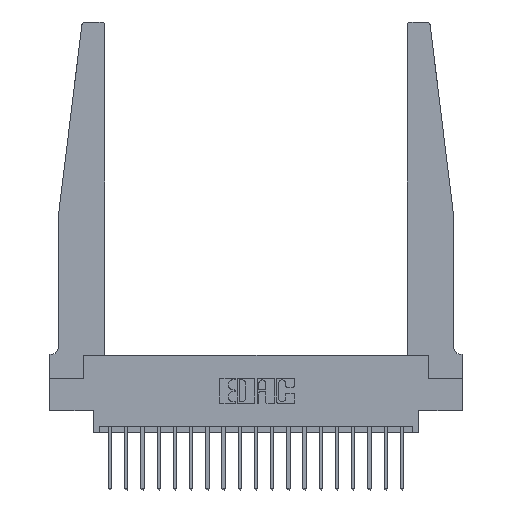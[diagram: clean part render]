
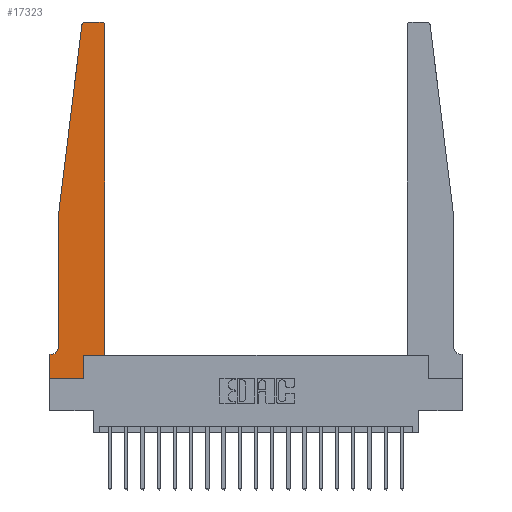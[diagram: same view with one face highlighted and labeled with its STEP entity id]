
A CAD part, top view. The second image highlights one B-rep face of the part: STEP entity #17323.
In plain terms, the highlighted planar face has unit normal (0, 0, 1).
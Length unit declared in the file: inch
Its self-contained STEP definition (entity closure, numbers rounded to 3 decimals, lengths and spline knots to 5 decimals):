
#47 = CARTESIAN_POINT ( 'NONE',  ( 0.2605, 0.18, 0.37 ) ) ;
#132 = VECTOR ( 'NONE', #20609, 39.37008 ) ;
#240 = LINE ( 'NONE', #17672, #7731 ) ;
#1497 = ORIENTED_EDGE ( 'NONE', *, *, #16786, .T. ) ;
#1586 = EDGE_CURVE ( 'NONE', #15586, #9109, #5750, .T. ) ;
#1587 = CARTESIAN_POINT ( 'NONE',  ( 0.27653, 2.72, 0.37 ) ) ;
#2582 = CARTESIAN_POINT ( 'NONE',  ( 0.065, 1.25, 0.37 ) ) ;
#2878 = VERTEX_POINT ( 'NONE', #9176 ) ;
#3000 = VERTEX_POINT ( 'NONE', #47 ) ;
#3519 = VECTOR ( 'NONE', #15939, 39.37008 ) ;
#3667 = CARTESIAN_POINT ( 'NONE',  ( 0.425, 2.72, 0.37 ) ) ;
#3804 = EDGE_CURVE ( 'NONE', #12323, #13643, #16821, .T. ) ;
#4185 = DIRECTION ( 'NONE',  ( 0., -1., 0. ) ) ;
#4323 = AXIS2_PLACEMENT_3D ( 'NONE', #16338, #6846, #18126 ) ;
#4395 = LINE ( 'NONE', #7848, #6207 ) ;
#4576 = VECTOR ( 'NONE', #19691, 39.37008 ) ;
#5034 = VECTOR ( 'NONE', #5542, 39.37008 ) ;
#5292 = ORIENTED_EDGE ( 'NONE', *, *, #1586, .T. ) ;
#5542 = DIRECTION ( 'NONE',  ( -0.122, -0.992, 0. ) ) ;
#5750 = CIRCLE ( 'NONE', #15189, 0.03 ) ;
#6018 = FACE_OUTER_BOUND ( 'NONE', #18411, .T. ) ;
#6207 = VECTOR ( 'NONE', #20681, 39.37008 ) ;
#6268 = ORIENTED_EDGE ( 'NONE', *, *, #15083, .T. ) ;
#6432 = EDGE_CURVE ( 'NONE', #2878, #19198, #14744, .T. ) ;
#6476 = CIRCLE ( 'NONE', #10875, 0.03 ) ;
#6534 = CARTESIAN_POINT ( 'NONE',  ( 0.425, 0.18, 0.37 ) ) ;
#6609 = DIRECTION ( 'NONE',  ( -1., 0., 0. ) ) ;
#6846 = DIRECTION ( 'NONE',  ( 0., 0., -1. ) ) ;
#6865 = LINE ( 'NONE', #19290, #10274 ) ;
#6880 = EDGE_CURVE ( 'NONE', #9109, #13700, #240, .T. ) ;
#6904 = EDGE_CURVE ( 'NONE', #13643, #2878, #16839, .T. ) ;
#6980 = CARTESIAN_POINT ( 'NONE',  ( 0., 0., 0.37 ) ) ;
#7018 = ORIENTED_EDGE ( 'NONE', *, *, #18342, .T. ) ;
#7120 = CARTESIAN_POINT ( 'NONE',  ( 0.065, 1.25, 0.37 ) ) ;
#7731 = VECTOR ( 'NONE', #6609, 39.37008 ) ;
#7848 = CARTESIAN_POINT ( 'NONE',  ( 0.2605, 0.18, 0.37 ) ) ;
#8049 = DIRECTION ( 'NONE',  ( 0., 0., 1. ) ) ;
#8143 = LINE ( 'NONE', #13001, #132 ) ;
#8332 = CARTESIAN_POINT ( 'NONE',  ( 0.395, 2.72, 0.37 ) ) ;
#8699 = ORIENTED_EDGE ( 'NONE', *, *, #3804, .T. ) ;
#8808 = EDGE_CURVE ( 'NONE', #13700, #12323, #6476, .T. ) ;
#8910 = CARTESIAN_POINT ( 'NONE',  ( 0.065, 1.25, 0.37 ) ) ;
#9109 = VERTEX_POINT ( 'NONE', #15541 ) ;
#9176 = CARTESIAN_POINT ( 'NONE',  ( 0.065, 0.2375, 0.37 ) ) ;
#9269 = CARTESIAN_POINT ( 'NONE',  ( 0., 0.1875, 0.37 ) ) ;
#9501 = CARTESIAN_POINT ( 'NONE',  ( 0.425, 0.18, 0.37 ) ) ;
#9592 = LINE ( 'NONE', #9501, #3519 ) ;
#10148 = DIRECTION ( 'NONE',  ( 0., -1., 0. ) ) ;
#10180 = ORIENTED_EDGE ( 'NONE', *, *, #8808, .T. ) ;
#10274 = VECTOR ( 'NONE', #14686, 39.37008 ) ;
#10875 = AXIS2_PLACEMENT_3D ( 'NONE', #1587, #8049, #11531 ) ;
#10895 = CARTESIAN_POINT ( 'NONE',  ( 0., 0., 0.37 ) ) ;
#11385 = EDGE_CURVE ( 'NONE', #3000, #20236, #19581, .T. ) ;
#11531 = DIRECTION ( 'NONE',  ( 1., 0., 0. ) ) ;
#11639 = VERTEX_POINT ( 'NONE', #12572 ) ;
#11799 = VECTOR ( 'NONE', #4185, 39.37008 ) ;
#11976 = ORIENTED_EDGE ( 'NONE', *, *, #16377, .T. ) ;
#12323 = VERTEX_POINT ( 'NONE', #19642 ) ;
#12463 = PLANE ( 'NONE',  #17398 ) ;
#12572 = CARTESIAN_POINT ( 'NONE',  ( 0., 0.1875, 0.37 ) ) ;
#12592 = ORIENTED_EDGE ( 'NONE', *, *, #11385, .T. ) ;
#13001 = CARTESIAN_POINT ( 'NONE',  ( 0., 0., 0.37 ) ) ;
#13522 = DIRECTION ( 'NONE',  ( 0., 0., 1. ) ) ;
#13526 = CARTESIAN_POINT ( 'NONE',  ( 0.2605, 0., 0.37 ) ) ;
#13643 = VERTEX_POINT ( 'NONE', #7120 ) ;
#13700 = VERTEX_POINT ( 'NONE', #15567 ) ;
#14534 = ORIENTED_EDGE ( 'NONE', *, *, #6432, .T. ) ;
#14686 = DIRECTION ( 'NONE',  ( -1., 0., 0. ) ) ;
#14744 = CIRCLE ( 'NONE', #4323, 0.05 ) ;
#14754 = CARTESIAN_POINT ( 'NONE',  ( 0.425, 0.18, 0.37 ) ) ;
#15083 = EDGE_CURVE ( 'NONE', #18611, #3000, #4395, .T. ) ;
#15189 = AXIS2_PLACEMENT_3D ( 'NONE', #8332, #13522, #18242 ) ;
#15541 = CARTESIAN_POINT ( 'NONE',  ( 0.395, 2.75, 0.37 ) ) ;
#15567 = CARTESIAN_POINT ( 'NONE',  ( 0.27653, 2.75, 0.37 ) ) ;
#15586 = VERTEX_POINT ( 'NONE', #3667 ) ;
#15939 = DIRECTION ( 'NONE',  ( 0., 1., 0. ) ) ;
#16329 = VECTOR ( 'NONE', #10148, 39.37008 ) ;
#16338 = CARTESIAN_POINT ( 'NONE',  ( 0.015, 0.2375, 0.37 ) ) ;
#16377 = EDGE_CURVE ( 'NONE', #18731, #18611, #8143, .T. ) ;
#16467 = EDGE_CURVE ( 'NONE', #11639, #18731, #18253, .T. ) ;
#16481 = ORIENTED_EDGE ( 'NONE', *, *, #16467, .T. ) ;
#16484 = ORIENTED_EDGE ( 'NONE', *, *, #6904, .T. ) ;
#16786 = EDGE_CURVE ( 'NONE', #20236, #15586, #9592, .T. ) ;
#16821 = LINE ( 'NONE', #8910, #5034 ) ;
#16839 = LINE ( 'NONE', #2582, #11799 ) ;
#17286 = CARTESIAN_POINT ( 'NONE',  ( 0.015, 0.1875, 0.37 ) ) ;
#17323 = ADVANCED_FACE ( 'NONE', ( #6018 ), #12463, .T. ) ;
#17391 = DIRECTION ( 'NONE',  ( 0., 0., 1. ) ) ;
#17398 = AXIS2_PLACEMENT_3D ( 'NONE', #9269, #17391, #20637 ) ;
#17672 = CARTESIAN_POINT ( 'NONE',  ( 0.25, 2.75, 0.37 ) ) ;
#18126 = DIRECTION ( 'NONE',  ( -1., 0., 0. ) ) ;
#18242 = DIRECTION ( 'NONE',  ( 1., 0., 0. ) ) ;
#18253 = LINE ( 'NONE', #6980, #16329 ) ;
#18342 = EDGE_CURVE ( 'NONE', #19198, #11639, #6865, .T. ) ;
#18411 = EDGE_LOOP ( 'NONE', ( #18706, #10180, #8699, #16484, #14534, #7018, #16481, #11976, #6268, #12592, #1497, #5292 ) ) ;
#18611 = VERTEX_POINT ( 'NONE', #13526 ) ;
#18706 = ORIENTED_EDGE ( 'NONE', *, *, #6880, .T. ) ;
#18731 = VERTEX_POINT ( 'NONE', #10895 ) ;
#19198 = VERTEX_POINT ( 'NONE', #17286 ) ;
#19290 = CARTESIAN_POINT ( 'NONE',  ( 0.065, 0.1875, 0.37 ) ) ;
#19581 = LINE ( 'NONE', #6534, #4576 ) ;
#19642 = CARTESIAN_POINT ( 'NONE',  ( 0.24675, 2.72367, 0.37 ) ) ;
#19691 = DIRECTION ( 'NONE',  ( 1., 0., 0. ) ) ;
#20236 = VERTEX_POINT ( 'NONE', #14754 ) ;
#20609 = DIRECTION ( 'NONE',  ( 1., 0., 0. ) ) ;
#20637 = DIRECTION ( 'NONE',  ( 1., 0., 0. ) ) ;
#20681 = DIRECTION ( 'NONE',  ( 0., 1., 0. ) ) ;
